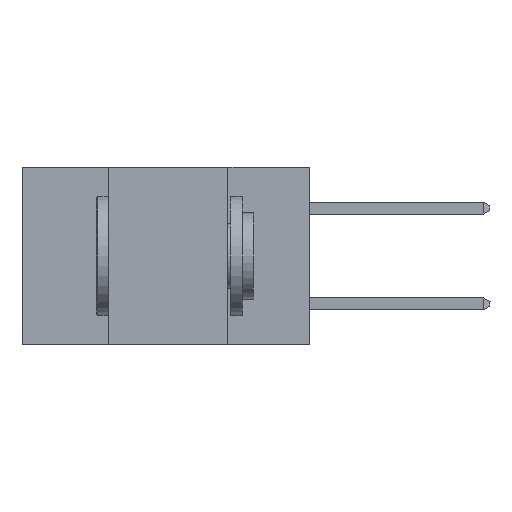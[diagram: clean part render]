
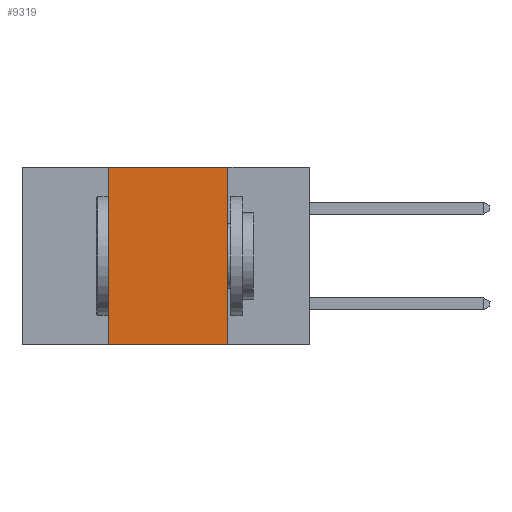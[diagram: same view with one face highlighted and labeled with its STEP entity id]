
A CAD part, left-side view. The second image highlights one B-rep face of the part: STEP entity #9319.
In plain terms, the highlighted planar face has unit normal (-1, 0, 0).
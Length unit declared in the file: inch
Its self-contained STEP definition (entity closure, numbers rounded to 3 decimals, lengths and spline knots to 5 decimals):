
#789 = EDGE_LOOP ( 'NONE', ( #12550, #12042, #9682, #3743 ) ) ;
#1500 = DIRECTION ( 'NONE',  ( 0., -1., 0. ) ) ;
#1669 = LINE ( 'NONE', #20044, #3402 ) ;
#3287 = CARTESIAN_POINT ( 'NONE',  ( 0., 0.17, -0.37 ) ) ;
#3402 = VECTOR ( 'NONE', #1500, 39.37008 ) ;
#3665 = DIRECTION ( 'NONE',  ( 0., -1., 0. ) ) ;
#3699 = CARTESIAN_POINT ( 'NONE',  ( 0., 0.42, 0. ) ) ;
#3743 = ORIENTED_EDGE ( 'NONE', *, *, #7423, .T. ) ;
#3907 = VERTEX_POINT ( 'NONE', #14179 ) ;
#5915 = VECTOR ( 'NONE', #16411, 39.37008 ) ;
#6573 = VERTEX_POINT ( 'NONE', #15829 ) ;
#6611 = EDGE_CURVE ( 'NONE', #6573, #3907, #1669, .T. ) ;
#6983 = FACE_OUTER_BOUND ( 'NONE', #789, .T. ) ;
#7116 = CARTESIAN_POINT ( 'NONE',  ( 0., 0.42, -0.37 ) ) ;
#7423 = EDGE_CURVE ( 'NONE', #11912, #26444, #25561, .T. ) ;
#8186 = LINE ( 'NONE', #16875, #9551 ) ;
#9319 = ADVANCED_FACE ( 'NONE', ( #6983 ), #21384, .F. ) ;
#9551 = VECTOR ( 'NONE', #21298, 39.37008 ) ;
#9682 = ORIENTED_EDGE ( 'NONE', *, *, #9947, .F. ) ;
#9947 = EDGE_CURVE ( 'NONE', #11912, #6573, #24804, .T. ) ;
#9950 = CARTESIAN_POINT ( 'NONE',  ( 0., 0.6, -0.37 ) ) ;
#10796 = EDGE_CURVE ( 'NONE', #3907, #26444, #8186, .T. ) ;
#10998 = DIRECTION ( 'NONE',  ( 0., 0., -1. ) ) ;
#11721 = VECTOR ( 'NONE', #3665, 39.37008 ) ;
#11912 = VERTEX_POINT ( 'NONE', #7116 ) ;
#12042 = ORIENTED_EDGE ( 'NONE', *, *, #6611, .F. ) ;
#12550 = ORIENTED_EDGE ( 'NONE', *, *, #10796, .F. ) ;
#14179 = CARTESIAN_POINT ( 'NONE',  ( 0., 0.17, 0. ) ) ;
#15232 = DIRECTION ( 'NONE',  ( 1., 0., 0. ) ) ;
#15829 = CARTESIAN_POINT ( 'NONE',  ( 0., 0.42, 0. ) ) ;
#16411 = DIRECTION ( 'NONE',  ( 0., 0., 1. ) ) ;
#16875 = CARTESIAN_POINT ( 'NONE',  ( 0., 0.17, 0. ) ) ;
#20044 = CARTESIAN_POINT ( 'NONE',  ( 0., 0.6, 0. ) ) ;
#21298 = DIRECTION ( 'NONE',  ( 0., 0., -1. ) ) ;
#21384 = PLANE ( 'NONE',  #27846 ) ;
#23948 = CARTESIAN_POINT ( 'NONE',  ( 0., 0.6, 0. ) ) ;
#24804 = LINE ( 'NONE', #3699, #5915 ) ;
#25561 = LINE ( 'NONE', #9950, #11721 ) ;
#26444 = VERTEX_POINT ( 'NONE', #3287 ) ;
#27846 = AXIS2_PLACEMENT_3D ( 'NONE', #23948, #15232, #10998 ) ;
